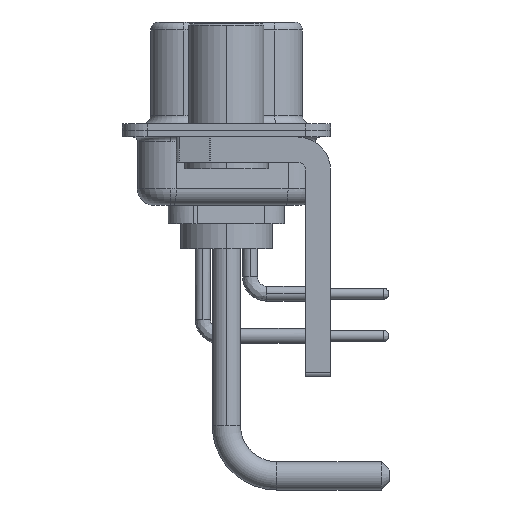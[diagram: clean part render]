
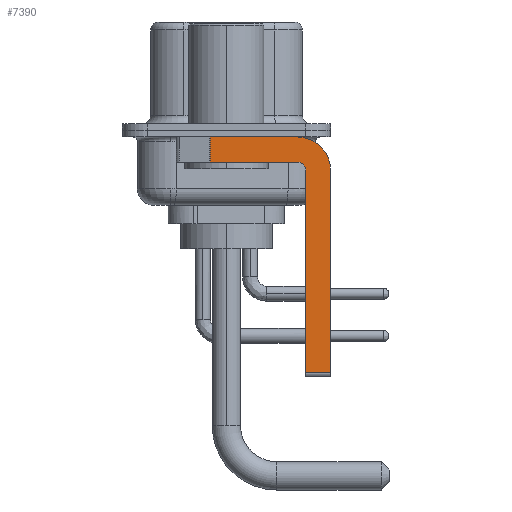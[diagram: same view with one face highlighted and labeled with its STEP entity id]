
A CAD part, left-side view. The second image highlights one B-rep face of the part: STEP entity #7390.
In plain terms, the highlighted planar face has unit normal (-1, 0, 0).
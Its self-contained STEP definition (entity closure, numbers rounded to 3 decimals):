
#165 = CIRCLE ( 'NONE', #19906, 0.5 ) ;
#220 = LINE ( 'NONE', #4019, #8543 ) ;
#399 = DIRECTION ( 'NONE',  ( 0., 0., 1. ) ) ;
#892 = DIRECTION ( 'NONE',  ( 0., 0., -1. ) ) ;
#972 = CARTESIAN_POINT ( 'NONE',  ( -2.9, -4.25, -1.9 ) ) ;
#979 = DIRECTION ( 'NONE',  ( 0., 0., 1. ) ) ;
#1149 = CARTESIAN_POINT ( 'NONE',  ( -2.9, -4.25, -1.9 ) ) ;
#1402 = CARTESIAN_POINT ( 'NONE',  ( -2.9, 3., -0.4 ) ) ;
#2545 = LINE ( 'NONE', #1149, #11480 ) ;
#2636 = CARTESIAN_POINT ( 'NONE',  ( -2.9, -4.25, -14.55 ) ) ;
#2874 = ORIENTED_EDGE ( 'NONE', *, *, #14179, .F. ) ;
#3693 = CIRCLE ( 'NONE', #13746, 2. ) ;
#4019 = CARTESIAN_POINT ( 'NONE',  ( -2.9, -6.25, -2.4 ) ) ;
#4467 = VECTOR ( 'NONE', #979, 1000. ) ;
#5563 = VERTEX_POINT ( 'NONE', #9543 ) ;
#5695 = DIRECTION ( 'NONE',  ( 0., -1., 0. ) ) ;
#5796 = ORIENTED_EDGE ( 'NONE', *, *, #21258, .T. ) ;
#6038 = DIRECTION ( 'NONE',  ( 0., 0., -1. ) ) ;
#7239 = CARTESIAN_POINT ( 'NONE',  ( -2.9, -4.25, -2.4 ) ) ;
#7390 = ADVANCED_FACE ( 'NONE', ( #16463 ), #24538, .F. ) ;
#7500 = VERTEX_POINT ( 'NONE', #11656 ) ;
#8543 = VECTOR ( 'NONE', #6038, 1000. ) ;
#8853 = LINE ( 'NONE', #20334, #23947 ) ;
#8886 = VERTEX_POINT ( 'NONE', #16950 ) ;
#9007 = CARTESIAN_POINT ( 'NONE',  ( -2.9, -4.25, -2.4 ) ) ;
#9543 = CARTESIAN_POINT ( 'NONE',  ( -2.9, -4.75, -2.4 ) ) ;
#9948 = VECTOR ( 'NONE', #10343, 1000. ) ;
#10322 = VECTOR ( 'NONE', #5695, 1000. ) ;
#10343 = DIRECTION ( 'NONE',  ( 0., -1., 0. ) ) ;
#10439 = VERTEX_POINT ( 'NONE', #20450 ) ;
#11187 = CARTESIAN_POINT ( 'NONE',  ( -2.9, 0.978, -1.9 ) ) ;
#11450 = EDGE_CURVE ( 'NONE', #5563, #21716, #165, .T. ) ;
#11480 = VECTOR ( 'NONE', #18328, 1000. ) ;
#11656 = CARTESIAN_POINT ( 'NONE',  ( -2.9, 0.978, -0.4 ) ) ;
#11777 = CARTESIAN_POINT ( 'NONE',  ( -2.9, -6.25, -2.4 ) ) ;
#12151 = ORIENTED_EDGE ( 'NONE', *, *, #13458, .F. ) ;
#12978 = ORIENTED_EDGE ( 'NONE', *, *, #11450, .F. ) ;
#13049 = DIRECTION ( 'NONE',  ( 0., 0., -1. ) ) ;
#13363 = VERTEX_POINT ( 'NONE', #14487 ) ;
#13458 = EDGE_CURVE ( 'NONE', #10439, #5563, #20037, .T. ) ;
#13653 = CARTESIAN_POINT ( 'NONE',  ( -2.9, -4.25, -2.4 ) ) ;
#13746 = AXIS2_PLACEMENT_3D ( 'NONE', #9007, #16701, #23138 ) ;
#14179 = EDGE_CURVE ( 'NONE', #8886, #22829, #3693, .T. ) ;
#14309 = ORIENTED_EDGE ( 'NONE', *, *, #18632, .T. ) ;
#14487 = CARTESIAN_POINT ( 'NONE',  ( -2.9, -6.25, -14.55 ) ) ;
#16037 = EDGE_LOOP ( 'NONE', ( #19296, #14309, #18087, #12978, #12151, #5796, #21333, #2874 ) ) ;
#16255 = CARTESIAN_POINT ( 'NONE',  ( -2.9, -4.75, -14.8 ) ) ;
#16411 = EDGE_CURVE ( 'NONE', #22829, #13363, #220, .T. ) ;
#16463 = FACE_OUTER_BOUND ( 'NONE', #16037, .T. ) ;
#16701 = DIRECTION ( 'NONE',  ( 1., 0., 0. ) ) ;
#16738 = VERTEX_POINT ( 'NONE', #11187 ) ;
#16950 = CARTESIAN_POINT ( 'NONE',  ( -2.9, -4.25, -0.4 ) ) ;
#17705 = DIRECTION ( 'NONE',  ( -1., 0., 0. ) ) ;
#18087 = ORIENTED_EDGE ( 'NONE', *, *, #19403, .F. ) ;
#18328 = DIRECTION ( 'NONE',  ( 0., 1., 0. ) ) ;
#18632 = EDGE_CURVE ( 'NONE', #7500, #16738, #8853, .T. ) ;
#18702 = LINE ( 'NONE', #1402, #10322 ) ;
#19296 = ORIENTED_EDGE ( 'NONE', *, *, #20923, .F. ) ;
#19403 = EDGE_CURVE ( 'NONE', #21716, #16738, #2545, .T. ) ;
#19906 = AXIS2_PLACEMENT_3D ( 'NONE', #13653, #17705, #399 ) ;
#20037 = LINE ( 'NONE', #16255, #4467 ) ;
#20334 = CARTESIAN_POINT ( 'NONE',  ( -2.9, 0.978, -1.9 ) ) ;
#20450 = CARTESIAN_POINT ( 'NONE',  ( -2.9, -4.75, -14.55 ) ) ;
#20611 = AXIS2_PLACEMENT_3D ( 'NONE', #7239, #24164, #13049 ) ;
#20923 = EDGE_CURVE ( 'NONE', #7500, #8886, #18702, .T. ) ;
#21258 = EDGE_CURVE ( 'NONE', #10439, #13363, #23973, .T. ) ;
#21333 = ORIENTED_EDGE ( 'NONE', *, *, #16411, .F. ) ;
#21716 = VERTEX_POINT ( 'NONE', #972 ) ;
#22829 = VERTEX_POINT ( 'NONE', #11777 ) ;
#23138 = DIRECTION ( 'NONE',  ( 0., 0., -1. ) ) ;
#23947 = VECTOR ( 'NONE', #892, 1000. ) ;
#23973 = LINE ( 'NONE', #2636, #9948 ) ;
#24164 = DIRECTION ( 'NONE',  ( 1., 0., 0. ) ) ;
#24538 = PLANE ( 'NONE',  #20611 ) ;
